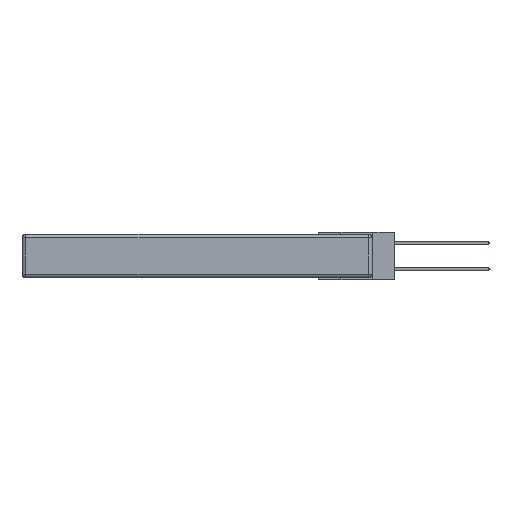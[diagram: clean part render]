
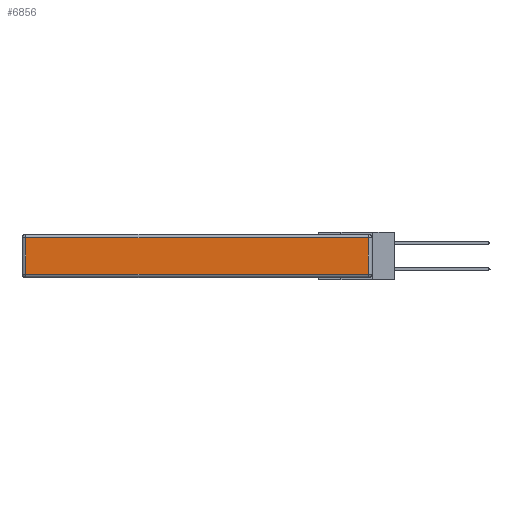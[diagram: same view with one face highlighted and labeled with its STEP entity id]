
A CAD part, left-side view. The second image highlights one B-rep face of the part: STEP entity #6856.
In plain terms, the highlighted planar face has unit normal (-1, 0, 0).
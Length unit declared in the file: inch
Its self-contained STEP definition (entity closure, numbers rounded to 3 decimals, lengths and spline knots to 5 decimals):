
#864 = EDGE_LOOP ( 'NONE', ( #5630, #2782, #19919, #30715 ) ) ;
#2509 = EDGE_CURVE ( 'NONE', #20586, #25581, #19180, .T. ) ;
#2782 = ORIENTED_EDGE ( 'NONE', *, *, #14998, .T. ) ;
#3358 = DIRECTION ( 'NONE',  ( 0., 0., 1. ) ) ;
#3710 = DIRECTION ( 'NONE',  ( -1., 0., 0. ) ) ;
#5630 = ORIENTED_EDGE ( 'NONE', *, *, #20011, .T. ) ;
#6485 = CARTESIAN_POINT ( 'NONE',  ( 0., 0., -0.313 ) ) ;
#6627 = VERTEX_POINT ( 'NONE', #34638 ) ;
#6856 = ADVANCED_FACE ( 'NONE', ( #25621 ), #34253, .T. ) ;
#8233 = VERTEX_POINT ( 'NONE', #27452 ) ;
#9682 = LINE ( 'NONE', #12636, #12292 ) ;
#10415 = LINE ( 'NONE', #6485, #22133 ) ;
#11338 = CARTESIAN_POINT ( 'NONE',  ( 0., 2.75, -0.03 ) ) ;
#11859 = CARTESIAN_POINT ( 'NONE',  ( 0., 0.03, -0.03 ) ) ;
#11886 = CARTESIAN_POINT ( 'NONE',  ( 0., 0., -0.343 ) ) ;
#12292 = VECTOR ( 'NONE', #18285, 39.37008 ) ;
#12636 = CARTESIAN_POINT ( 'NONE',  ( 0., 2.72, -0.343 ) ) ;
#14998 = EDGE_CURVE ( 'NONE', #8233, #20586, #15624, .T. ) ;
#15624 = LINE ( 'NONE', #34447, #32503 ) ;
#16129 = VECTOR ( 'NONE', #22334, 39.37008 ) ;
#18285 = DIRECTION ( 'NONE',  ( 0., 0., -1. ) ) ;
#18562 = AXIS2_PLACEMENT_3D ( 'NONE', #11886, #3710, #3358 ) ;
#19180 = LINE ( 'NONE', #11338, #16129 ) ;
#19919 = ORIENTED_EDGE ( 'NONE', *, *, #2509, .T. ) ;
#20011 = EDGE_CURVE ( 'NONE', #6627, #8233, #10415, .T. ) ;
#20446 = DIRECTION ( 'NONE',  ( 0., -1., 0. ) ) ;
#20586 = VERTEX_POINT ( 'NONE', #11859 ) ;
#22133 = VECTOR ( 'NONE', #20446, 39.37008 ) ;
#22334 = DIRECTION ( 'NONE',  ( 0., 1., 0. ) ) ;
#23633 = CARTESIAN_POINT ( 'NONE',  ( 0., 2.72, -0.03 ) ) ;
#25581 = VERTEX_POINT ( 'NONE', #23633 ) ;
#25621 = FACE_OUTER_BOUND ( 'NONE', #864, .T. ) ;
#27452 = CARTESIAN_POINT ( 'NONE',  ( 0., 0.03, -0.313 ) ) ;
#30715 = ORIENTED_EDGE ( 'NONE', *, *, #33274, .T. ) ;
#31528 = DIRECTION ( 'NONE',  ( 0., 0., 1. ) ) ;
#32503 = VECTOR ( 'NONE', #31528, 39.37008 ) ;
#33274 = EDGE_CURVE ( 'NONE', #25581, #6627, #9682, .T. ) ;
#34253 = PLANE ( 'NONE',  #18562 ) ;
#34447 = CARTESIAN_POINT ( 'NONE',  ( 0., 0.03, -0.343 ) ) ;
#34638 = CARTESIAN_POINT ( 'NONE',  ( 0., 2.72, -0.313 ) ) ;
